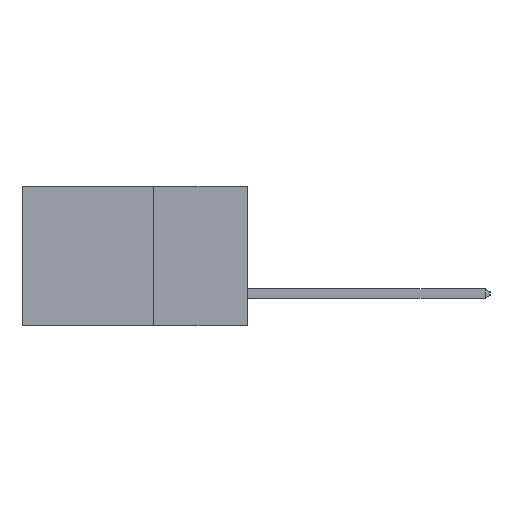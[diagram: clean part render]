
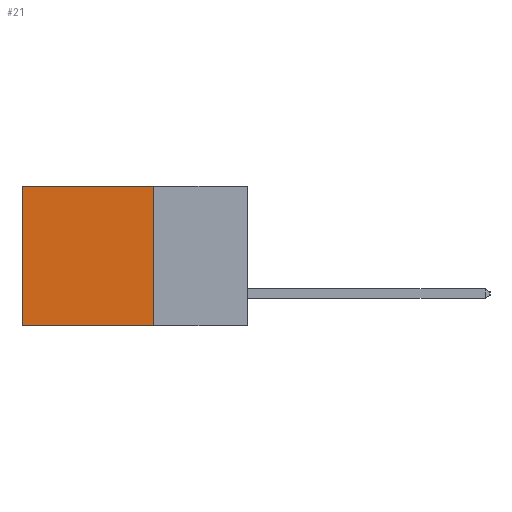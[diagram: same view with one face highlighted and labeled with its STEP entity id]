
A CAD part, left-side view. The second image highlights one B-rep face of the part: STEP entity #21.
In plain terms, the highlighted planar face has unit normal (-1, 0, 0).
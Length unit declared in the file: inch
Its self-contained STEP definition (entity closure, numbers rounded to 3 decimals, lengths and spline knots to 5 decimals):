
#21 = ADVANCED_FACE ( 'NONE', ( #13769 ), #3853, .F. ) ;
#141 = CARTESIAN_POINT ( 'NONE',  ( 0.2615, 0.6, -0.37 ) ) ;
#303 = CARTESIAN_POINT ( 'NONE',  ( 0.2615, 0.6, 0. ) ) ;
#454 = LINE ( 'NONE', #10277, #1241 ) ;
#959 = DIRECTION ( 'NONE',  ( 0., 1., 0. ) ) ;
#1009 = LINE ( 'NONE', #11451, #3116 ) ;
#1170 = DIRECTION ( 'NONE',  ( 1., 0., 0. ) ) ;
#1241 = VECTOR ( 'NONE', #11422, 39.37008 ) ;
#2217 = EDGE_LOOP ( 'NONE', ( #7185, #8149, #8420, #8496 ) ) ;
#2402 = VECTOR ( 'NONE', #6979, 39.37008 ) ;
#3116 = VECTOR ( 'NONE', #11579, 39.37008 ) ;
#3670 = EDGE_CURVE ( 'NONE', #10288, #5698, #14334, .T. ) ;
#3853 = PLANE ( 'NONE',  #5582 ) ;
#4833 = EDGE_CURVE ( 'NONE', #4984, #5273, #1009, .T. ) ;
#4984 = VERTEX_POINT ( 'NONE', #14159 ) ;
#5273 = VERTEX_POINT ( 'NONE', #5659 ) ;
#5582 = AXIS2_PLACEMENT_3D ( 'NONE', #11863, #1170, #7315 ) ;
#5659 = CARTESIAN_POINT ( 'NONE',  ( 0.2615, 0.25, -0.37 ) ) ;
#5698 = VERTEX_POINT ( 'NONE', #141 ) ;
#6809 = CARTESIAN_POINT ( 'NONE',  ( 0.2615, 0.6, -0.37 ) ) ;
#6920 = CARTESIAN_POINT ( 'NONE',  ( 0.2615, 0.25, 0. ) ) ;
#6979 = DIRECTION ( 'NONE',  ( 0., 0., -1. ) ) ;
#7185 = ORIENTED_EDGE ( 'NONE', *, *, #3670, .T. ) ;
#7315 = DIRECTION ( 'NONE',  ( 0., 0., -1. ) ) ;
#7649 = LINE ( 'NONE', #6920, #13366 ) ;
#8149 = ORIENTED_EDGE ( 'NONE', *, *, #13559, .F. ) ;
#8420 = ORIENTED_EDGE ( 'NONE', *, *, #4833, .F. ) ;
#8496 = ORIENTED_EDGE ( 'NONE', *, *, #10593, .T. ) ;
#10277 = CARTESIAN_POINT ( 'NONE',  ( 0.2615, 0.25, -0.37 ) ) ;
#10288 = VERTEX_POINT ( 'NONE', #303 ) ;
#10593 = EDGE_CURVE ( 'NONE', #4984, #10288, #7649, .T. ) ;
#11422 = DIRECTION ( 'NONE',  ( 0., 1., 0. ) ) ;
#11451 = CARTESIAN_POINT ( 'NONE',  ( 0.2615, 0.25, -0.37 ) ) ;
#11579 = DIRECTION ( 'NONE',  ( 0., 0., -1. ) ) ;
#11863 = CARTESIAN_POINT ( 'NONE',  ( 0.2615, 0.25, -0.37 ) ) ;
#13366 = VECTOR ( 'NONE', #959, 39.37008 ) ;
#13559 = EDGE_CURVE ( 'NONE', #5273, #5698, #454, .T. ) ;
#13769 = FACE_OUTER_BOUND ( 'NONE', #2217, .T. ) ;
#14159 = CARTESIAN_POINT ( 'NONE',  ( 0.2615, 0.25, 0. ) ) ;
#14334 = LINE ( 'NONE', #6809, #2402 ) ;
